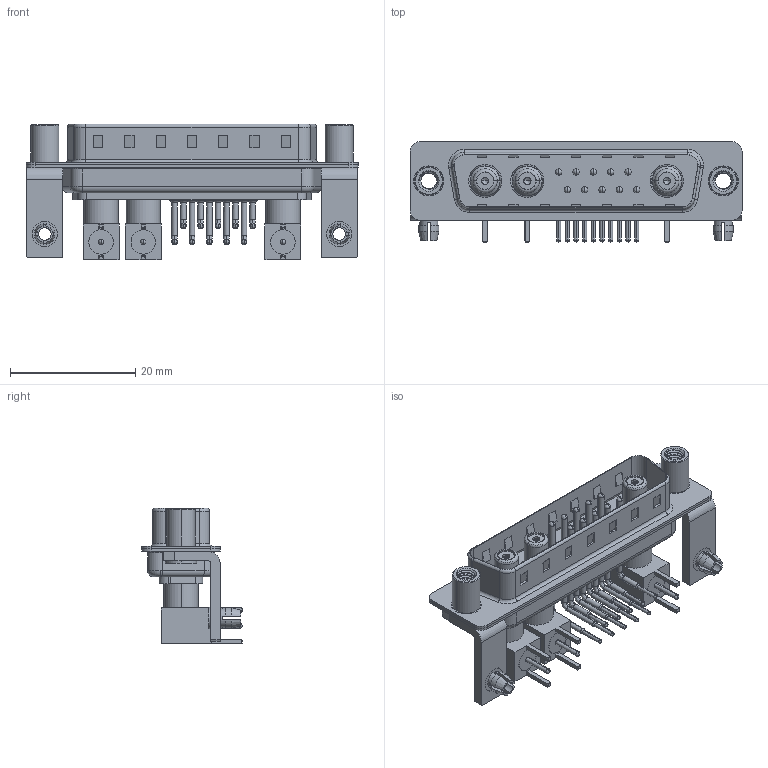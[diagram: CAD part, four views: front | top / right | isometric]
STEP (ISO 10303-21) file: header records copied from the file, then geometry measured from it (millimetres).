
FILE_DESCRIPTION (( 'STEP AP203' ), '1' );
FILE_NAME ('629-13W3240-7TD.STEP', '2022-05-10T03:00:48', ( '' ), ( '' ), 'SwSTEP 2.0', 'SolidWorks 2020', '' );
FILE_SCHEMA (( 'CONFIG_CONTROL_DESIGN' ));
Length unit declared in the file: millimetre
Products named in the file (19): Co-Ax Jack_RA PC Tail; Insulator Socket 2; 629Combo Threaded Standoff_D; 629Combo Board Lock; Co-Ax Jack Assy_RA; Socket_RA; RA Back Shell; Insulator RA Pin; 629Combo Contact Row 2; Locking Collar; 629Combo Shell Rear_25 Contacts; 629Combo Contact Row 1; Insulator Socket; 629Combo Housing_13W3; 629Combo Stabilizer Bracket; 629Combo Shell Front_25 Contacts; 629-13W3240-7TD
Assembly tree (43 placements, depth 3):
  629-13W3240-7TD
    629Combo Housing_13W3
    629Combo Shell Rear_25 Contacts
    629Combo Shell Front_25 Contacts
    629Combo Stabilizer Bracket  x2
    629Combo Board Lock  x2
    629Combo Threaded Standoff_D  x2
    Co-Ax Jack Assy_RA
      Co-Ax Jack_RA PC Tail
      Insulator Socket
      Insulator Socket 2
      Locking Collar
      Socket_RA
      RA Back Shell
      Insulator RA Pin
    Co-Ax Jack Assy_RA
      Co-Ax Jack_RA PC Tail
      Insulator Socket
      Insulator Socket 2
      Locking Collar
      Socket_RA
      RA Back Shell
      Insulator RA Pin
    Co-Ax Jack Assy_RA
      Co-Ax Jack_RA PC Tail
      Insulator Socket
      Insulator Socket 2
      Locking Collar
      Socket_RA
      RA Back Shell
      Insulator RA Pin
    629Combo Contact Row 1  x5
    629Combo Contact Row 2  x5
Bounding box: 53.05 x 16 x 21.71 mm (x, y, z)
Volume: 4074.8 mm3; surface area: 11039.3 mm2
Topology: 40 solids, 40 shells, 2122 faces, 5616 edges, 3609 vertices
Faces by surface type: plane 1052, cylinder 802, cone 125, bspline 69, torus 68, sphere 6
Entity records: 32176 total; most frequent: CARTESIAN_POINT 7444, DIRECTION 4784, ORIENTED_EDGE 4496, EDGE_CURVE 2248, AXIS2_PLACEMENT_3D 1735, VERTEX_POINT 1448, LINE 1314, VECTOR 1314
